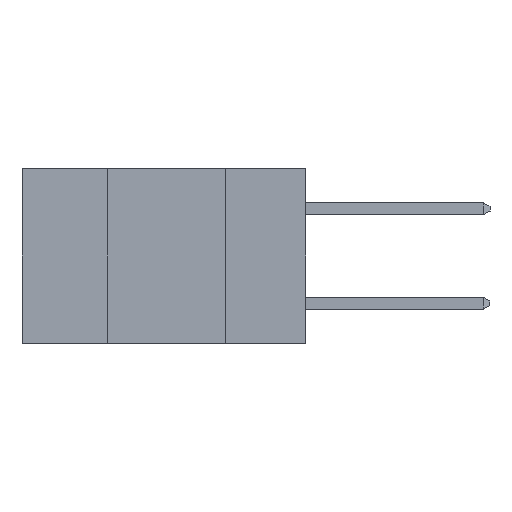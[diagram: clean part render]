
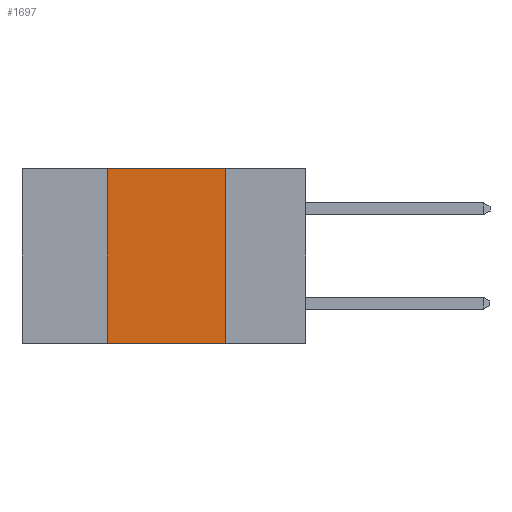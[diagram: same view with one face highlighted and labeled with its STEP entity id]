
A CAD part, left-side view. The second image highlights one B-rep face of the part: STEP entity #1697.
In plain terms, the highlighted planar face has unit normal (-1, 0, 0).
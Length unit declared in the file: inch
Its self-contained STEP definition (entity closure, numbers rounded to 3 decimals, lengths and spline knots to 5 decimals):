
#148 = VERTEX_POINT ( 'NONE', #11373 ) ;
#364 = VERTEX_POINT ( 'NONE', #4182 ) ;
#496 = VERTEX_POINT ( 'NONE', #4894 ) ;
#1697 = ADVANCED_FACE ( 'NONE', ( #6572 ), #10256, .F. ) ;
#2027 = CARTESIAN_POINT ( 'NONE',  ( 0., 0.42, -0.37 ) ) ;
#2386 = CARTESIAN_POINT ( 'NONE',  ( 0., 0.17, 0. ) ) ;
#2666 = ORIENTED_EDGE ( 'NONE', *, *, #10268, .F. ) ;
#3099 = VERTEX_POINT ( 'NONE', #2027 ) ;
#3292 = VECTOR ( 'NONE', #9329, 39.37008 ) ;
#3810 = LINE ( 'NONE', #7398, #10790 ) ;
#4022 = DIRECTION ( 'NONE',  ( 0., 0., -1. ) ) ;
#4182 = CARTESIAN_POINT ( 'NONE',  ( 0., 0.17, -0.37 ) ) ;
#4271 = DIRECTION ( 'NONE',  ( 0., 0., -1. ) ) ;
#4894 = CARTESIAN_POINT ( 'NONE',  ( 0., 0.17, 0. ) ) ;
#5200 = VECTOR ( 'NONE', #10257, 39.37008 ) ;
#5815 = VECTOR ( 'NONE', #4271, 39.37008 ) ;
#6253 = CARTESIAN_POINT ( 'NONE',  ( 0., 0.6, 0. ) ) ;
#6328 = EDGE_CURVE ( 'NONE', #148, #496, #3810, .T. ) ;
#6572 = FACE_OUTER_BOUND ( 'NONE', #8092, .T. ) ;
#7398 = CARTESIAN_POINT ( 'NONE',  ( 0., 0.6, 0. ) ) ;
#7559 = CARTESIAN_POINT ( 'NONE',  ( 0., 0.42, 0. ) ) ;
#7720 = LINE ( 'NONE', #9797, #5200 ) ;
#7987 = LINE ( 'NONE', #7559, #3292 ) ;
#8092 = EDGE_LOOP ( 'NONE', ( #2666, #11337, #10512, #11465 ) ) ;
#9164 = DIRECTION ( 'NONE',  ( 0., -1., 0. ) ) ;
#9329 = DIRECTION ( 'NONE',  ( 0., 0., 1. ) ) ;
#9668 = DIRECTION ( 'NONE',  ( 1., 0., 0. ) ) ;
#9797 = CARTESIAN_POINT ( 'NONE',  ( 0., 0.6, -0.37 ) ) ;
#9996 = AXIS2_PLACEMENT_3D ( 'NONE', #6253, #9668, #4022 ) ;
#10256 = PLANE ( 'NONE',  #9996 ) ;
#10257 = DIRECTION ( 'NONE',  ( 0., -1., 0. ) ) ;
#10268 = EDGE_CURVE ( 'NONE', #496, #364, #10608, .T. ) ;
#10299 = EDGE_CURVE ( 'NONE', #3099, #148, #7987, .T. ) ;
#10341 = EDGE_CURVE ( 'NONE', #3099, #364, #7720, .T. ) ;
#10512 = ORIENTED_EDGE ( 'NONE', *, *, #10299, .F. ) ;
#10608 = LINE ( 'NONE', #2386, #5815 ) ;
#10790 = VECTOR ( 'NONE', #9164, 39.37008 ) ;
#11337 = ORIENTED_EDGE ( 'NONE', *, *, #6328, .F. ) ;
#11373 = CARTESIAN_POINT ( 'NONE',  ( 0., 0.42, 0. ) ) ;
#11465 = ORIENTED_EDGE ( 'NONE', *, *, #10341, .T. ) ;
